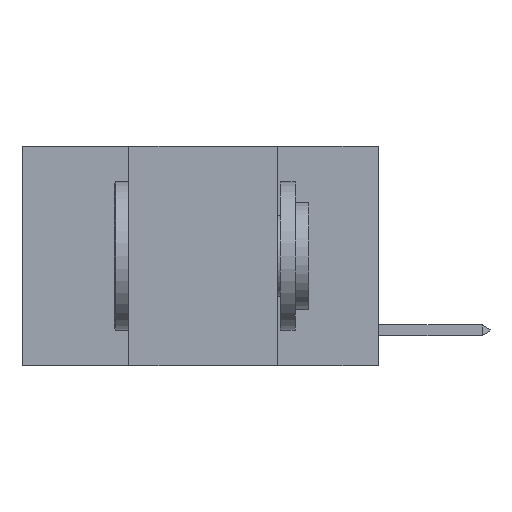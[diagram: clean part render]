
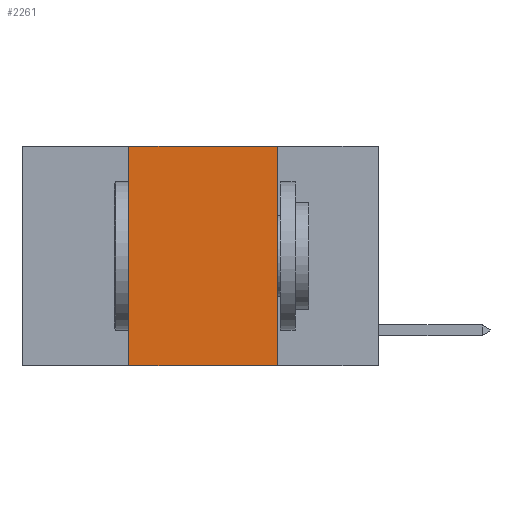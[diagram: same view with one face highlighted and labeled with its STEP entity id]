
A CAD part, left-side view. The second image highlights one B-rep face of the part: STEP entity #2261.
In plain terms, the highlighted planar face has unit normal (-1, 0, 0).
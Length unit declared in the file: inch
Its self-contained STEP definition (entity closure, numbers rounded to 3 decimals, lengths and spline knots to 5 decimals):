
#5 = VERTEX_POINT ( 'NONE', #14863 ) ;
#306 = CARTESIAN_POINT ( 'NONE',  ( 0., 0.6, 0. ) ) ;
#496 = ORIENTED_EDGE ( 'NONE', *, *, #6445, .T. ) ;
#663 = EDGE_CURVE ( 'NONE', #4692, #17835, #15824, .T. ) ;
#2261 = ADVANCED_FACE ( 'NONE', ( #6883 ), #5874, .F. ) ;
#2507 = LINE ( 'NONE', #306, #11484 ) ;
#3205 = VECTOR ( 'NONE', #17955, 39.37008 ) ;
#3375 = CARTESIAN_POINT ( 'NONE',  ( 0., 0.42, 0. ) ) ;
#4287 = CARTESIAN_POINT ( 'NONE',  ( 0., 0.42, -0.37 ) ) ;
#4692 = VERTEX_POINT ( 'NONE', #4287 ) ;
#5027 = AXIS2_PLACEMENT_3D ( 'NONE', #13446, #7344, #11686 ) ;
#5874 = PLANE ( 'NONE',  #5027 ) ;
#6124 = VECTOR ( 'NONE', #9915, 39.37008 ) ;
#6445 = EDGE_CURVE ( 'NONE', #4692, #17231, #14934, .T. ) ;
#6567 = DIRECTION ( 'NONE',  ( 0., -1., 0. ) ) ;
#6883 = FACE_OUTER_BOUND ( 'NONE', #13065, .T. ) ;
#7237 = ORIENTED_EDGE ( 'NONE', *, *, #16597, .F. ) ;
#7344 = DIRECTION ( 'NONE',  ( 1., 0., 0. ) ) ;
#8468 = ORIENTED_EDGE ( 'NONE', *, *, #15253, .F. ) ;
#8547 = CARTESIAN_POINT ( 'NONE',  ( 0., 0.42, 0. ) ) ;
#9456 = ORIENTED_EDGE ( 'NONE', *, *, #663, .F. ) ;
#9915 = DIRECTION ( 'NONE',  ( 0., 0., -1. ) ) ;
#11484 = VECTOR ( 'NONE', #6567, 39.37008 ) ;
#11495 = CARTESIAN_POINT ( 'NONE',  ( 0., 0.6, -0.37 ) ) ;
#11686 = DIRECTION ( 'NONE',  ( 0., 0., -1. ) ) ;
#13061 = CARTESIAN_POINT ( 'NONE',  ( 0., 0.17, 0. ) ) ;
#13065 = EDGE_LOOP ( 'NONE', ( #7237, #8468, #9456, #496 ) ) ;
#13446 = CARTESIAN_POINT ( 'NONE',  ( 0., 0.6, 0. ) ) ;
#14586 = CARTESIAN_POINT ( 'NONE',  ( 0., 0.17, -0.37 ) ) ;
#14863 = CARTESIAN_POINT ( 'NONE',  ( 0., 0.17, 0. ) ) ;
#14934 = LINE ( 'NONE', #11495, #17467 ) ;
#15096 = LINE ( 'NONE', #13061, #6124 ) ;
#15253 = EDGE_CURVE ( 'NONE', #17835, #5, #2507, .T. ) ;
#15824 = LINE ( 'NONE', #8547, #3205 ) ;
#16085 = DIRECTION ( 'NONE',  ( 0., -1., 0. ) ) ;
#16597 = EDGE_CURVE ( 'NONE', #5, #17231, #15096, .T. ) ;
#17231 = VERTEX_POINT ( 'NONE', #14586 ) ;
#17467 = VECTOR ( 'NONE', #16085, 39.37008 ) ;
#17835 = VERTEX_POINT ( 'NONE', #3375 ) ;
#17955 = DIRECTION ( 'NONE',  ( 0., 0., 1. ) ) ;
